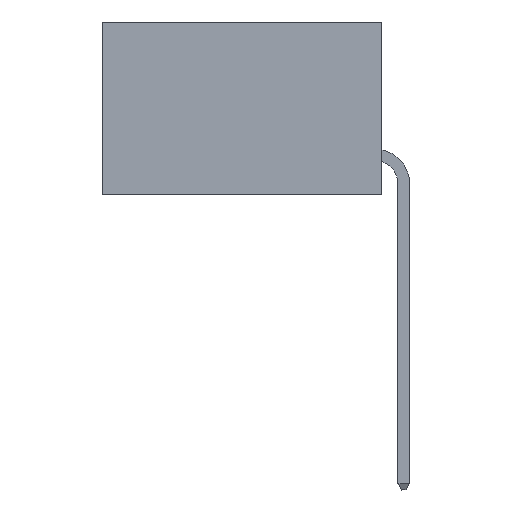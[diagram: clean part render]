
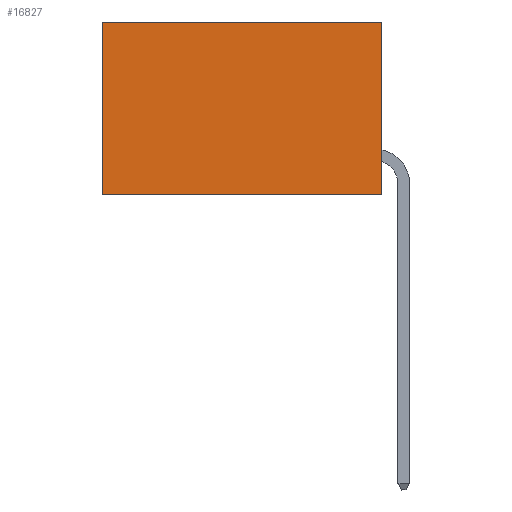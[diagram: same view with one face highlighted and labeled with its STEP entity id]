
A CAD part, left-side view. The second image highlights one B-rep face of the part: STEP entity #16827.
In plain terms, the highlighted planar face has unit normal (-1, 0, 0).
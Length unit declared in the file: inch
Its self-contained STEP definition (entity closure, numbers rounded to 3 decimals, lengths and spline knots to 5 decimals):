
#1224 = ORIENTED_EDGE ( 'NONE', *, *, #26402, .F. ) ;
#1829 = ORIENTED_EDGE ( 'NONE', *, *, #9524, .T. ) ;
#2092 = ORIENTED_EDGE ( 'NONE', *, *, #5086, .T. ) ;
#3751 = DIRECTION ( 'NONE',  ( 0., 1., 0. ) ) ;
#5086 = EDGE_CURVE ( 'NONE', #8550, #30469, #6316, .T. ) ;
#6116 = CARTESIAN_POINT ( 'NONE',  ( 0.2875, 0., 0. ) ) ;
#6205 = LINE ( 'NONE', #22051, #6642 ) ;
#6316 = LINE ( 'NONE', #23300, #33244 ) ;
#6413 = DIRECTION ( 'NONE',  ( 0., 0., -1. ) ) ;
#6642 = VECTOR ( 'NONE', #6413, 39.37008 ) ;
#7499 = DIRECTION ( 'NONE',  ( 0., 1., 0. ) ) ;
#7680 = DIRECTION ( 'NONE',  ( 0., 0., -1. ) ) ;
#8550 = VERTEX_POINT ( 'NONE', #21382 ) ;
#8691 = VERTEX_POINT ( 'NONE', #22033 ) ;
#9524 = EDGE_CURVE ( 'NONE', #8691, #8550, #20363, .T. ) ;
#10585 = CARTESIAN_POINT ( 'NONE',  ( 0.2875, 0., -0.37 ) ) ;
#10833 = VECTOR ( 'NONE', #7499, 39.37008 ) ;
#11409 = DIRECTION ( 'NONE',  ( 1., 0., 0. ) ) ;
#13230 = ORIENTED_EDGE ( 'NONE', *, *, #25571, .F. ) ;
#13856 = CARTESIAN_POINT ( 'NONE',  ( 0.2875, 0., 0. ) ) ;
#14453 = VERTEX_POINT ( 'NONE', #30923 ) ;
#15116 = CARTESIAN_POINT ( 'NONE',  ( 0.2875, 0.6, -0.37 ) ) ;
#15525 = AXIS2_PLACEMENT_3D ( 'NONE', #6116, #11409, #16439 ) ;
#16439 = DIRECTION ( 'NONE',  ( 0., 0., -1. ) ) ;
#16827 = ADVANCED_FACE ( 'NONE', ( #18933 ), #21779, .F. ) ;
#18933 = FACE_OUTER_BOUND ( 'NONE', #33208, .T. ) ;
#20363 = LINE ( 'NONE', #13856, #30885 ) ;
#21382 = CARTESIAN_POINT ( 'NONE',  ( 0.2875, 0.6, 0. ) ) ;
#21779 = PLANE ( 'NONE',  #15525 ) ;
#22033 = CARTESIAN_POINT ( 'NONE',  ( 0.2875, 0., 0. ) ) ;
#22051 = CARTESIAN_POINT ( 'NONE',  ( 0.2875, 0., 0. ) ) ;
#23049 = LINE ( 'NONE', #10585, #10833 ) ;
#23300 = CARTESIAN_POINT ( 'NONE',  ( 0.2875, 0.6, 0. ) ) ;
#25571 = EDGE_CURVE ( 'NONE', #14453, #30469, #23049, .T. ) ;
#26402 = EDGE_CURVE ( 'NONE', #8691, #14453, #6205, .T. ) ;
#30469 = VERTEX_POINT ( 'NONE', #15116 ) ;
#30885 = VECTOR ( 'NONE', #3751, 39.37008 ) ;
#30923 = CARTESIAN_POINT ( 'NONE',  ( 0.2875, 0., -0.37 ) ) ;
#33208 = EDGE_LOOP ( 'NONE', ( #2092, #13230, #1224, #1829 ) ) ;
#33244 = VECTOR ( 'NONE', #7680, 39.37008 ) ;
